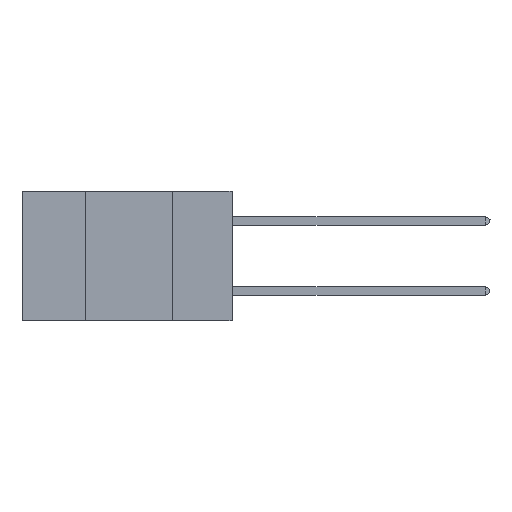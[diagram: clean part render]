
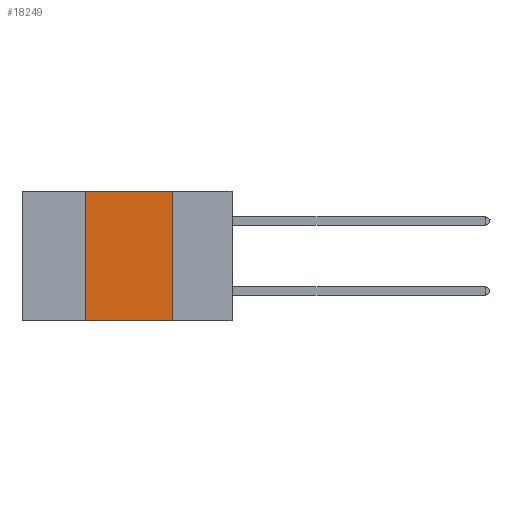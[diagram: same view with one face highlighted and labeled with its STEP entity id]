
A CAD part, left-side view. The second image highlights one B-rep face of the part: STEP entity #18249.
In plain terms, the highlighted planar face has unit normal (-1, 0, 0).
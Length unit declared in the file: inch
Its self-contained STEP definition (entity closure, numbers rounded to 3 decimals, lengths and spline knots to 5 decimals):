
#452 = CARTESIAN_POINT ( 'NONE',  ( 0., 0.17, 0. ) ) ;
#1272 = LINE ( 'NONE', #10918, #25340 ) ;
#1648 = VERTEX_POINT ( 'NONE', #18080 ) ;
#4321 = VECTOR ( 'NONE', #17336, 39.37008 ) ;
#5676 = CARTESIAN_POINT ( 'NONE',  ( 0., 0.6, 0. ) ) ;
#8201 = ORIENTED_EDGE ( 'NONE', *, *, #18024, .F. ) ;
#8271 = ORIENTED_EDGE ( 'NONE', *, *, #13212, .F. ) ;
#8849 = CARTESIAN_POINT ( 'NONE',  ( 0., 0.42, 0. ) ) ;
#8935 = VERTEX_POINT ( 'NONE', #30792 ) ;
#9764 = LINE ( 'NONE', #452, #31742 ) ;
#10918 = CARTESIAN_POINT ( 'NONE',  ( 0., 0.42, 0. ) ) ;
#11575 = VERTEX_POINT ( 'NONE', #8849 ) ;
#13139 = DIRECTION ( 'NONE',  ( 0., -1., 0. ) ) ;
#13203 = VERTEX_POINT ( 'NONE', #18367 ) ;
#13212 = EDGE_CURVE ( 'NONE', #8935, #13203, #9764, .T. ) ;
#16434 = DIRECTION ( 'NONE',  ( 0., 0., -1. ) ) ;
#17336 = DIRECTION ( 'NONE',  ( 0., -1., 0. ) ) ;
#18024 = EDGE_CURVE ( 'NONE', #11575, #8935, #25100, .T. ) ;
#18080 = CARTESIAN_POINT ( 'NONE',  ( 0., 0.42, -0.37 ) ) ;
#18249 = ADVANCED_FACE ( 'NONE', ( #31471 ), #32627, .F. ) ;
#18323 = ORIENTED_EDGE ( 'NONE', *, *, #30750, .T. ) ;
#18336 = CARTESIAN_POINT ( 'NONE',  ( 0., 0.6, 0. ) ) ;
#18367 = CARTESIAN_POINT ( 'NONE',  ( 0., 0.17, -0.37 ) ) ;
#19129 = DIRECTION ( 'NONE',  ( 0., 0., -1. ) ) ;
#20332 = EDGE_CURVE ( 'NONE', #1648, #11575, #1272, .T. ) ;
#21452 = AXIS2_PLACEMENT_3D ( 'NONE', #5676, #32864, #19129 ) ;
#21699 = VECTOR ( 'NONE', #13139, 39.37008 ) ;
#25100 = LINE ( 'NONE', #18336, #21699 ) ;
#25340 = VECTOR ( 'NONE', #27209, 39.37008 ) ;
#25381 = CARTESIAN_POINT ( 'NONE',  ( 0., 0.6, -0.37 ) ) ;
#26002 = ORIENTED_EDGE ( 'NONE', *, *, #20332, .F. ) ;
#27209 = DIRECTION ( 'NONE',  ( 0., 0., 1. ) ) ;
#30060 = EDGE_LOOP ( 'NONE', ( #8271, #8201, #26002, #18323 ) ) ;
#30517 = LINE ( 'NONE', #25381, #4321 ) ;
#30750 = EDGE_CURVE ( 'NONE', #1648, #13203, #30517, .T. ) ;
#30792 = CARTESIAN_POINT ( 'NONE',  ( 0., 0.17, 0. ) ) ;
#31471 = FACE_OUTER_BOUND ( 'NONE', #30060, .T. ) ;
#31742 = VECTOR ( 'NONE', #16434, 39.37008 ) ;
#32627 = PLANE ( 'NONE',  #21452 ) ;
#32864 = DIRECTION ( 'NONE',  ( 1., 0., 0. ) ) ;
